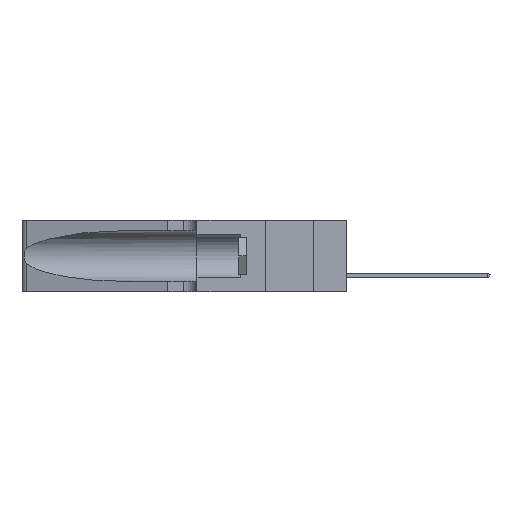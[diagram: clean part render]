
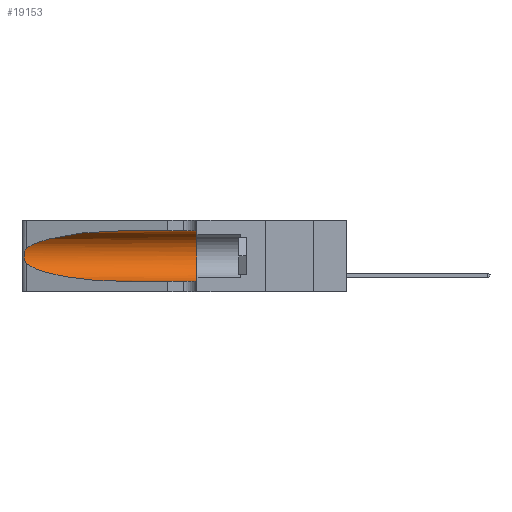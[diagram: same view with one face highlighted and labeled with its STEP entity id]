
A CAD part, left-side view. The second image highlights one B-rep face of the part: STEP entity #19153.
In plain terms, the highlighted cylindrical face has radius 3.308 mm (diameter 6.617 mm), a partial arc.
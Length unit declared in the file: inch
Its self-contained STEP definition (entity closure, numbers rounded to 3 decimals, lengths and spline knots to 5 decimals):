
#269 = VECTOR ( 'NONE', #6485, 39.37008 ) ;
#2514 = CARTESIAN_POINT ( 'NONE',  ( 0.1305, 0.72297, 0.05475 ) ) ;
#2863 = CARTESIAN_POINT ( 'NONE',  ( 0.2373, 1.15595, 0.28018 ) ) ;
#3000 = ORIENTED_EDGE ( 'NONE', *, *, #32228, .F. ) ;
#3248 = CARTESIAN_POINT ( 'NONE',  ( 0.25856, 1.23593, 0.16098 ) ) ;
#3532 = DIRECTION ( 'NONE',  ( 0., -1., 0. ) ) ;
#5369 = VECTOR ( 'NONE', #3532, 39.37008 ) ;
#6485 = DIRECTION ( 'NONE',  ( 0., -1., 0. ) ) ;
#6708 = CARTESIAN_POINT ( 'NONE',  ( 0.1305, 0.72297, 0.31525 ) ) ;
#7153 = CARTESIAN_POINT ( 'NONE',  ( 0.1305, 0.35, 0.185 ) ) ;
#8829 =( BOUNDED_CURVE ( )  B_SPLINE_CURVE ( 3, ( #14102, #31234, #2863, #23160 ),
 .UNSPECIFIED., .F., .F. ) 
 B_SPLINE_CURVE_WITH_KNOTS ( ( 4, 4 ),
 ( 1.5708, 2.84003 ),
 .UNSPECIFIED. ) 
 CURVE ( )  GEOMETRIC_REPRESENTATION_ITEM ( )  RATIONAL_B_SPLINE_CURVE ( ( 1., 0.87, 0.87, 1. ) ) 
 REPRESENTATION_ITEM ( '' )  );
#9496 = AXIS2_PLACEMENT_3D ( 'NONE', #9928, #30223, #15731 ) ;
#9928 = CARTESIAN_POINT ( 'NONE',  ( 0.1305, 1.61858, 0.185 ) ) ;
#9988 = AXIS2_PLACEMENT_3D ( 'NONE', #7153, #10308, #36134 ) ;
#10308 = DIRECTION ( 'NONE',  ( 0., 1., 0. ) ) ;
#10796 = ORIENTED_EDGE ( 'NONE', *, *, #27965, .F. ) ;
#10876 = VERTEX_POINT ( 'NONE', #19641 ) ;
#11054 = CARTESIAN_POINT ( 'NONE',  ( 0.25487, 1.22718, 0.14631 ) ) ;
#11743 = EDGE_CURVE ( 'NONE', #15552, #37367, #8829, .T. ) ;
#13030 = CARTESIAN_POINT ( 'NONE',  ( 0.25854, 1.2359, 0.20912 ) ) ;
#14102 = CARTESIAN_POINT ( 'NONE',  ( 0.1305, 0.72297, 0.31525 ) ) ;
#14315 = CARTESIAN_POINT ( 'NONE',  ( 0.25555, 1.22993, 0.14849 ) ) ;
#14343 = CARTESIAN_POINT ( 'NONE',  ( 0.2373, 1.15595, 0.08982 ) ) ;
#14368 = ORIENTED_EDGE ( 'NONE', *, *, #37215, .T. ) ;
#14663 = ORIENTED_EDGE ( 'NONE', *, *, #30657, .T. ) ;
#15113 = CARTESIAN_POINT ( 'NONE',  ( 0.1305, 1.61858, 0.05475 ) ) ;
#15552 = VERTEX_POINT ( 'NONE', #6708 ) ;
#15731 = DIRECTION ( 'NONE',  ( 0., 0., -1. ) ) ;
#16683 = CARTESIAN_POINT ( 'NONE',  ( 0.26017, 1.23833, 0.17102 ) ) ;
#17342 = CIRCLE ( 'NONE', #9988, 0.13025 ) ;
#19153 = ADVANCED_FACE ( 'NONE', ( #19370 ), #20246, .F. ) ;
#19370 = FACE_OUTER_BOUND ( 'NONE', #25513, .T. ) ;
#19641 = CARTESIAN_POINT ( 'NONE',  ( 0.1305, 0.35, 0.31525 ) ) ;
#20137 = CARTESIAN_POINT ( 'NONE',  ( 0.25487, 1.22718, 0.14631 ) ) ;
#20174 = VERTEX_POINT ( 'NONE', #29523 ) ;
#20246 = CYLINDRICAL_SURFACE ( 'NONE', #9496, 0.13025 ) ;
#21756 = CARTESIAN_POINT ( 'NONE',  ( 0.25787, 1.23484, 0.2124 ) ) ;
#21920 = VERTEX_POINT ( 'NONE', #36450 ) ;
#22284 = B_SPLINE_CURVE_WITH_KNOTS ( 'NONE', 3,
 ( #32266, #32649, #28148, #21756, #13030, #29228, #23232, #25330, #16683, #3248, #35463, #30973, #14315, #11054 ),
 .UNSPECIFIED., .F., .F.,
 ( 4, 2, 2, 2, 2, 2, 4 ),
 ( 0., 0.00027, 0.00053, 0.00107, 0.0016, 0.00187, 0.00214 ),
 .UNSPECIFIED. ) ;
#22387 = ORIENTED_EDGE ( 'NONE', *, *, #28054, .T. ) ;
#23160 = CARTESIAN_POINT ( 'NONE',  ( 0.25487, 1.22718, 0.22369 ) ) ;
#23232 = CARTESIAN_POINT ( 'NONE',  ( 0.26075, 1.23896, 0.19203 ) ) ;
#23285 = LINE ( 'NONE', #35727, #269 ) ;
#23676 = CARTESIAN_POINT ( 'NONE',  ( 0.25487, 1.22718, 0.22369 ) ) ;
#24065 = VERTEX_POINT ( 'NONE', #26423 ) ;
#25240 = ORIENTED_EDGE ( 'NONE', *, *, #11743, .T. ) ;
#25330 = CARTESIAN_POINT ( 'NONE',  ( 0.26075, 1.23896, 0.178 ) ) ;
#25513 = EDGE_LOOP ( 'NONE', ( #25240, #14663, #14368, #22387, #3000, #10796 ) ) ;
#25780 = CARTESIAN_POINT ( 'NONE',  ( 0.18966, 0.96281, 0.05475 ) ) ;
#26246 =( BOUNDED_CURVE ( )  B_SPLINE_CURVE ( 3, ( #20137, #14343, #25780, #2514 ),
 .UNSPECIFIED., .F., .F. ) 
 B_SPLINE_CURVE_WITH_KNOTS ( ( 4, 4 ),
 ( 3.44316, 4.71239 ),
 .UNSPECIFIED. ) 
 CURVE ( )  GEOMETRIC_REPRESENTATION_ITEM ( )  RATIONAL_B_SPLINE_CURVE ( ( 1., 0.87, 0.87, 1. ) ) 
 REPRESENTATION_ITEM ( '' )  );
#26423 = CARTESIAN_POINT ( 'NONE',  ( 0.1305, 0.35, 0.05475 ) ) ;
#27965 = EDGE_CURVE ( 'NONE', #15552, #10876, #23285, .T. ) ;
#28054 = EDGE_CURVE ( 'NONE', #21920, #24065, #36628, .T. ) ;
#28148 = CARTESIAN_POINT ( 'NONE',  ( 0.25639, 1.23184, 0.21858 ) ) ;
#29228 = CARTESIAN_POINT ( 'NONE',  ( 0.26018, 1.23835, 0.19895 ) ) ;
#29523 = CARTESIAN_POINT ( 'NONE',  ( 0.25487, 1.22718, 0.14631 ) ) ;
#30223 = DIRECTION ( 'NONE',  ( 0., -1., 0. ) ) ;
#30657 = EDGE_CURVE ( 'NONE', #37367, #20174, #22284, .T. ) ;
#30973 = CARTESIAN_POINT ( 'NONE',  ( 0.25639, 1.23186, 0.15144 ) ) ;
#31234 = CARTESIAN_POINT ( 'NONE',  ( 0.18966, 0.96281, 0.31525 ) ) ;
#32228 = EDGE_CURVE ( 'NONE', #10876, #24065, #17342, .T. ) ;
#32266 = CARTESIAN_POINT ( 'NONE',  ( 0.25487, 1.22718, 0.22369 ) ) ;
#32649 = CARTESIAN_POINT ( 'NONE',  ( 0.25555, 1.22994, 0.2215 ) ) ;
#35463 = CARTESIAN_POINT ( 'NONE',  ( 0.25789, 1.23486, 0.15765 ) ) ;
#35727 = CARTESIAN_POINT ( 'NONE',  ( 0.1305, 1.61858, 0.31525 ) ) ;
#36134 = DIRECTION ( 'NONE',  ( 0., 0., 1. ) ) ;
#36450 = CARTESIAN_POINT ( 'NONE',  ( 0.1305, 0.72297, 0.05475 ) ) ;
#36628 = LINE ( 'NONE', #15113, #5369 ) ;
#37215 = EDGE_CURVE ( 'NONE', #20174, #21920, #26246, .T. ) ;
#37367 = VERTEX_POINT ( 'NONE', #23676 ) ;
